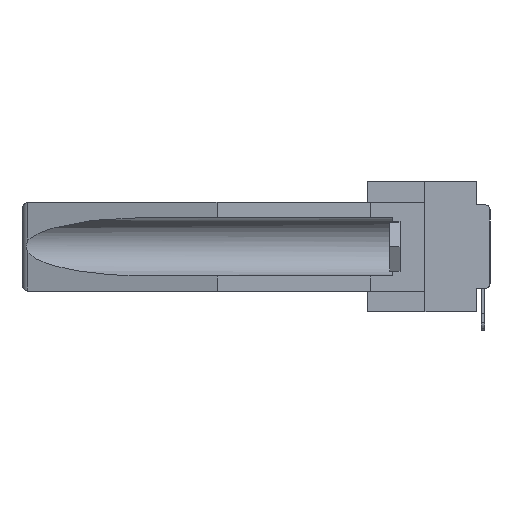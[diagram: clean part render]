
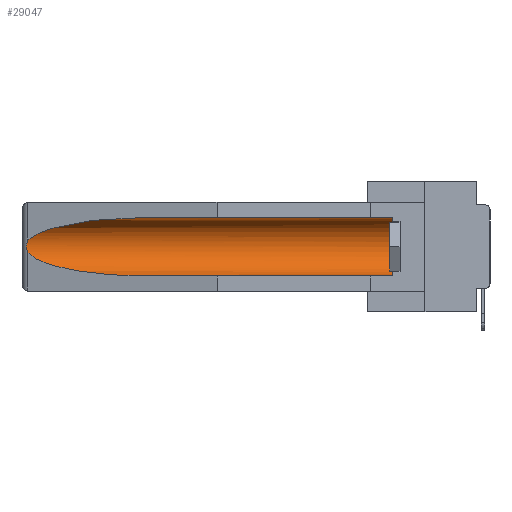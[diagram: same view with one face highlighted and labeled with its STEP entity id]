
A CAD part, left-side view. The second image highlights one B-rep face of the part: STEP entity #29047.
In plain terms, the highlighted cylindrical face has radius 2.857 mm (diameter 5.715 mm), a partial arc.
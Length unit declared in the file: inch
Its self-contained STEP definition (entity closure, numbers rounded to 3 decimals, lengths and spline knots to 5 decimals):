
#578 = CARTESIAN_POINT ( 'NONE',  ( 0.155, -0.30754, -0.1715 ) ) ;
#1875 = ORIENTED_EDGE ( 'NONE', *, *, #5805, .T. ) ;
#4165 = CARTESIAN_POINT ( 'NONE',  ( 0.2673, 1.53269, -0.17917 ) ) ;
#4230 = DIRECTION ( 'NONE',  ( 0., 0., 1. ) ) ;
#4554 = CARTESIAN_POINT ( 'NONE',  ( 0.21114, 1.30732, -0.059 ) ) ;
#4852 = VERTEX_POINT ( 'NONE', #34611 ) ;
#4985 = VECTOR ( 'NONE', #26019, 39.37008 ) ;
#5012 = ORIENTED_EDGE ( 'NONE', *, *, #9210, .F. ) ;
#5805 = EDGE_CURVE ( 'NONE', #22659, #19940, #22734, .T. ) ;
#5960 =( BOUNDED_CURVE ( )  B_SPLINE_CURVE ( 3, ( #37486, #11546, #35364, #8289 ),
 .UNSPECIFIED., .F., .F. ) 
 B_SPLINE_CURVE_WITH_KNOTS ( ( 4, 4 ),
 ( 0.1948, 1.5708 ),
 .UNSPECIFIED. ) 
 CURVE ( )  GEOMETRIC_REPRESENTATION_ITEM ( )  RATIONAL_B_SPLINE_CURVE ( ( 1., 0.848, 0.848, 1. ) ) 
 REPRESENTATION_ITEM ( '' )  );
#6522 = CYLINDRICAL_SURFACE ( 'NONE', #37525, 0.1125 ) ;
#7829 = CARTESIAN_POINT ( 'NONE',  ( 0.155, 1.07973, -0.059 ) ) ;
#8289 = CARTESIAN_POINT ( 'NONE',  ( 0.155, 1.07973, -0.284 ) ) ;
#8355 = LINE ( 'NONE', #28891, #4985 ) ;
#9192 = DIRECTION ( 'NONE',  ( 0., -1., 0. ) ) ;
#9210 = EDGE_CURVE ( 'NONE', #22659, #34149, #8355, .T. ) ;
#10234 = CARTESIAN_POINT ( 'NONE',  ( 0.26537, 1.52718, -0.19328 ) ) ;
#10752 = LINE ( 'NONE', #22082, #16576 ) ;
#11364 = EDGE_LOOP ( 'NONE', ( #11932, #11883, #30175, #5012, #1875, #33135 ) ) ;
#11546 = CARTESIAN_POINT ( 'NONE',  ( 0.25451, 1.48313, -0.24835 ) ) ;
#11883 = ORIENTED_EDGE ( 'NONE', *, *, #30945, .T. ) ;
#11932 = ORIENTED_EDGE ( 'NONE', *, *, #27642, .T. ) ;
#12635 = CARTESIAN_POINT ( 'NONE',  ( 0.155, 0.126, -0.1715 ) ) ;
#16576 = VECTOR ( 'NONE', #31289, 39.37008 ) ;
#16904 = CARTESIAN_POINT ( 'NONE',  ( 0.155, 1.07973, -0.059 ) ) ;
#16979 = CARTESIAN_POINT ( 'NONE',  ( 0.155, 0.126, -0.059 ) ) ;
#18234 = DIRECTION ( 'NONE',  ( 0., 1., 0. ) ) ;
#18791 = DIRECTION ( 'NONE',  ( 0., 0., 1. ) ) ;
#18922 = CARTESIAN_POINT ( 'NONE',  ( 0.2675, 1.53308, -0.17534 ) ) ;
#19940 = VERTEX_POINT ( 'NONE', #16979 ) ;
#21686 = FACE_OUTER_BOUND ( 'NONE', #11364, .T. ) ;
#21991 = CARTESIAN_POINT ( 'NONE',  ( 0.26537, 1.52718, -0.14972 ) ) ;
#22082 = CARTESIAN_POINT ( 'NONE',  ( 0.155, -0.30754, -0.059 ) ) ;
#22659 = VERTEX_POINT ( 'NONE', #31166 ) ;
#22734 = CIRCLE ( 'NONE', #27651, 0.1125 ) ;
#25245 = CARTESIAN_POINT ( 'NONE',  ( 0.2673, 1.5327, -0.16383 ) ) ;
#25491 = VERTEX_POINT ( 'NONE', #10234 ) ;
#26019 = DIRECTION ( 'NONE',  ( 0., 1., 0. ) ) ;
#27080 = EDGE_CURVE ( 'NONE', #25491, #34149, #5960, .T. ) ;
#27454 = EDGE_CURVE ( 'NONE', #19940, #31775, #10752, .T. ) ;
#27642 = EDGE_CURVE ( 'NONE', #31775, #4852, #29729, .T. ) ;
#27651 = AXIS2_PLACEMENT_3D ( 'NONE', #12635, #9192, #18791 ) ;
#27944 = CARTESIAN_POINT ( 'NONE',  ( 0.26537, 1.52718, -0.19328 ) ) ;
#28891 = CARTESIAN_POINT ( 'NONE',  ( 0.155, -0.30754, -0.284 ) ) ;
#29047 = ADVANCED_FACE ( 'NONE', ( #21686 ), #6522, .F. ) ;
#29316 = CARTESIAN_POINT ( 'NONE',  ( 0.155, 1.07973, -0.284 ) ) ;
#29729 =( BOUNDED_CURVE ( )  B_SPLINE_CURVE ( 3, ( #16904, #4554, #33527, #30265 ),
 .UNSPECIFIED., .F., .F. ) 
 B_SPLINE_CURVE_WITH_KNOTS ( ( 4, 4 ),
 ( 4.71239, 6.08839 ),
 .UNSPECIFIED. ) 
 CURVE ( )  GEOMETRIC_REPRESENTATION_ITEM ( )  RATIONAL_B_SPLINE_CURVE ( ( 1., 0.848, 0.848, 1. ) ) 
 REPRESENTATION_ITEM ( '' )  );
#30175 = ORIENTED_EDGE ( 'NONE', *, *, #27080, .T. ) ;
#30265 = CARTESIAN_POINT ( 'NONE',  ( 0.26537, 1.52718, -0.14972 ) ) ;
#30435 = CARTESIAN_POINT ( 'NONE',  ( 0.26597, 1.52961, -0.15275 ) ) ;
#30816 = CARTESIAN_POINT ( 'NONE',  ( 0.2675, 1.53308, -0.16763 ) ) ;
#30945 = EDGE_CURVE ( 'NONE', #4852, #25491, #37948, .T. ) ;
#31166 = CARTESIAN_POINT ( 'NONE',  ( 0.155, 0.126, -0.284 ) ) ;
#31289 = DIRECTION ( 'NONE',  ( 0., 1., 0. ) ) ;
#31775 = VERTEX_POINT ( 'NONE', #7829 ) ;
#33135 = ORIENTED_EDGE ( 'NONE', *, *, #27454, .T. ) ;
#33527 = CARTESIAN_POINT ( 'NONE',  ( 0.25451, 1.48313, -0.09465 ) ) ;
#33890 = CARTESIAN_POINT ( 'NONE',  ( 0.26597, 1.5296, -0.19026 ) ) ;
#34149 = VERTEX_POINT ( 'NONE', #29316 ) ;
#34611 = CARTESIAN_POINT ( 'NONE',  ( 0.26537, 1.52718, -0.14972 ) ) ;
#35364 = CARTESIAN_POINT ( 'NONE',  ( 0.21114, 1.30732, -0.284 ) ) ;
#36586 = CARTESIAN_POINT ( 'NONE',  ( 0.26654, 1.53092, -0.15636 ) ) ;
#36774 = CARTESIAN_POINT ( 'NONE',  ( 0.26655, 1.53094, -0.18657 ) ) ;
#37486 = CARTESIAN_POINT ( 'NONE',  ( 0.26537, 1.52718, -0.19328 ) ) ;
#37525 = AXIS2_PLACEMENT_3D ( 'NONE', #578, #18234, #4230 ) ;
#37948 = B_SPLINE_CURVE_WITH_KNOTS ( 'NONE', 3,
 ( #21991, #30435, #36586, #25245, #30816, #18922, #4165, #36774, #33890, #27944 ),
 .UNSPECIFIED., .F., .F.,
 ( 4, 2, 2, 2, 4 ),
 ( 0., 0.00029, 0.00058, 0.00087, 0.00117 ),
 .UNSPECIFIED. ) ;
